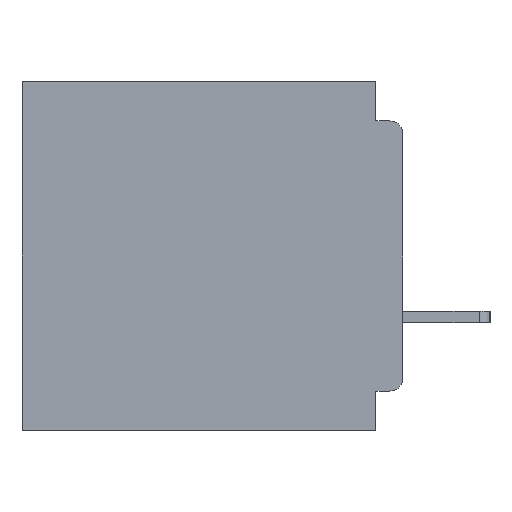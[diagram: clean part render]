
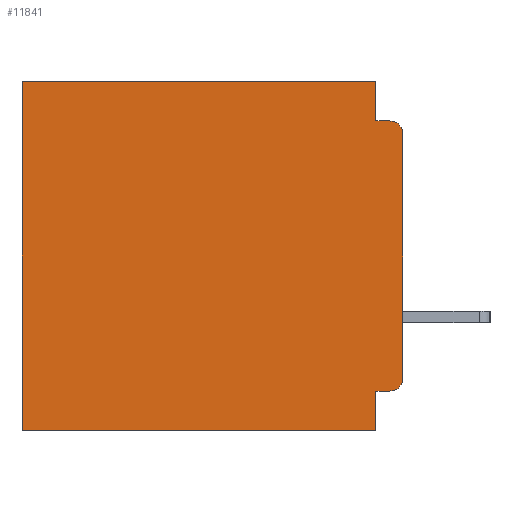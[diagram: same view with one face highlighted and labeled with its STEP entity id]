
A CAD part, left-side view. The second image highlights one B-rep face of the part: STEP entity #11841.
In plain terms, the highlighted planar face has unit normal (-1, 0, 0).
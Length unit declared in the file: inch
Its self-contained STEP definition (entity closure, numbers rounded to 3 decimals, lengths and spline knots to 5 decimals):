
#1046 = LINE ( 'NONE', #38750, #51141 ) ;
#1846 = CARTESIAN_POINT ( 'NONE',  ( 0.3, 0., -0.34 ) ) ;
#1952 = VERTEX_POINT ( 'NONE', #1846 ) ;
#2390 = ORIENTED_EDGE ( 'NONE', *, *, #43696, .T. ) ;
#2711 = ORIENTED_EDGE ( 'NONE', *, *, #8843, .F. ) ;
#3593 = VECTOR ( 'NONE', #11787, 39.37008 ) ;
#4501 = ORIENTED_EDGE ( 'NONE', *, *, #10820, .F. ) ;
#4968 = VERTEX_POINT ( 'NONE', #35830 ) ;
#4974 = EDGE_CURVE ( 'NONE', #32501, #1952, #7253, .T. ) ;
#5276 = ORIENTED_EDGE ( 'NONE', *, *, #4974, .F. ) ;
#5565 = CARTESIAN_POINT ( 'NONE',  ( 0.3, 0.031, -0.4 ) ) ;
#7253 = LINE ( 'NONE', #8095, #28355 ) ;
#7737 = CARTESIAN_POINT ( 'NONE',  ( 0.3, 0., -0.355 ) ) ;
#8095 = CARTESIAN_POINT ( 'NONE',  ( 0.3, 0., -0.4 ) ) ;
#8452 = EDGE_CURVE ( 'NONE', #32501, #28695, #13776, .T. ) ;
#8843 = EDGE_CURVE ( 'NONE', #15329, #44103, #26704, .T. ) ;
#9590 = CARTESIAN_POINT ( 'NONE',  ( 0.3, 0.437, -0.4 ) ) ;
#9704 = DIRECTION ( 'NONE',  ( 0., 1., 0. ) ) ;
#9792 = ORIENTED_EDGE ( 'NONE', *, *, #42569, .T. ) ;
#10611 = DIRECTION ( 'NONE',  ( 0., -1., 0. ) ) ;
#10820 = EDGE_CURVE ( 'NONE', #35454, #15329, #28352, .T. ) ;
#11787 = DIRECTION ( 'NONE',  ( 0., 1., 0. ) ) ;
#11841 = ADVANCED_FACE ( 'NONE', ( #50920 ), #15832, .F. ) ;
#12145 = DIRECTION ( 'NONE',  ( 0., 0., -1. ) ) ;
#13776 = CIRCLE ( 'NONE', #24136, 0.015 ) ;
#14290 = CIRCLE ( 'NONE', #14782, 0.015 ) ;
#14482 = DIRECTION ( 'NONE',  ( -1., 0., 0. ) ) ;
#14782 = AXIS2_PLACEMENT_3D ( 'NONE', #38891, #15288, #42840 ) ;
#14791 = ORIENTED_EDGE ( 'NONE', *, *, #27732, .F. ) ;
#14882 = EDGE_CURVE ( 'NONE', #40064, #35454, #35280, .T. ) ;
#15288 = DIRECTION ( 'NONE',  ( -1., 0., 0. ) ) ;
#15329 = VERTEX_POINT ( 'NONE', #18006 ) ;
#15335 = VECTOR ( 'NONE', #9704, 39.37008 ) ;
#15832 = PLANE ( 'NONE',  #17653 ) ;
#16653 = VECTOR ( 'NONE', #25360, 39.37008 ) ;
#17495 = VECTOR ( 'NONE', #40599, 39.37008 ) ;
#17653 = AXIS2_PLACEMENT_3D ( 'NONE', #27513, #51171, #27692 ) ;
#18006 = CARTESIAN_POINT ( 'NONE',  ( 0.3, 0.031, -0.4 ) ) ;
#19764 = ORIENTED_EDGE ( 'NONE', *, *, #47376, .F. ) ;
#19780 = CARTESIAN_POINT ( 'NONE',  ( 0.3, 0.031, -0.355 ) ) ;
#20289 = LINE ( 'NONE', #32781, #38764 ) ;
#24136 = AXIS2_PLACEMENT_3D ( 'NONE', #38087, #14482, #42040 ) ;
#25360 = DIRECTION ( 'NONE',  ( 0., 0., -1. ) ) ;
#26319 = ORIENTED_EDGE ( 'NONE', *, *, #14882, .F. ) ;
#26677 = EDGE_LOOP ( 'NONE', ( #5276, #44292, #14791, #19764, #9792, #2390, #2711, #4501, #26319, #32527 ) ) ;
#26704 = LINE ( 'NONE', #36692, #17495 ) ;
#26763 = LINE ( 'NONE', #42014, #45208 ) ;
#27513 = CARTESIAN_POINT ( 'NONE',  ( 0.3, 0., -0.4 ) ) ;
#27692 = DIRECTION ( 'NONE',  ( 0., 0., -1. ) ) ;
#27732 = EDGE_CURVE ( 'NONE', #4968, #28695, #26763, .T. ) ;
#28352 = LINE ( 'NONE', #5565, #16653 ) ;
#28355 = VECTOR ( 'NONE', #12145, 39.37008 ) ;
#28695 = VERTEX_POINT ( 'NONE', #32836 ) ;
#29425 = CARTESIAN_POINT ( 'NONE',  ( 0.3, 0., 0. ) ) ;
#30719 = VERTEX_POINT ( 'NONE', #50224 ) ;
#32501 = VERTEX_POINT ( 'NONE', #41996 ) ;
#32527 = ORIENTED_EDGE ( 'NONE', *, *, #33553, .T. ) ;
#32781 = CARTESIAN_POINT ( 'NONE',  ( 0.3, 0.437, -0.4 ) ) ;
#32836 = CARTESIAN_POINT ( 'NONE',  ( 0.3, 0.015, -0.045 ) ) ;
#33553 = EDGE_CURVE ( 'NONE', #40064, #1952, #14290, .T. ) ;
#35280 = LINE ( 'NONE', #7737, #3593 ) ;
#35454 = VERTEX_POINT ( 'NONE', #19780 ) ;
#35830 = CARTESIAN_POINT ( 'NONE',  ( 0.3, 0.031, -0.045 ) ) ;
#35983 = CARTESIAN_POINT ( 'NONE',  ( 0.3, 0.015, -0.355 ) ) ;
#36230 = VERTEX_POINT ( 'NONE', #36917 ) ;
#36321 = LINE ( 'NONE', #29425, #15335 ) ;
#36692 = CARTESIAN_POINT ( 'NONE',  ( 0.3, 0., -0.4 ) ) ;
#36917 = CARTESIAN_POINT ( 'NONE',  ( 0.3, 0.437, 0. ) ) ;
#38087 = CARTESIAN_POINT ( 'NONE',  ( 0.3, 0.015, -0.06 ) ) ;
#38750 = CARTESIAN_POINT ( 'NONE',  ( 0.3, 0.031, 0. ) ) ;
#38764 = VECTOR ( 'NONE', #48380, 39.37008 ) ;
#38891 = CARTESIAN_POINT ( 'NONE',  ( 0.3, 0.015, -0.34 ) ) ;
#40064 = VERTEX_POINT ( 'NONE', #35983 ) ;
#40599 = DIRECTION ( 'NONE',  ( 0., 1., 0. ) ) ;
#41996 = CARTESIAN_POINT ( 'NONE',  ( 0.3, 0., -0.06 ) ) ;
#42014 = CARTESIAN_POINT ( 'NONE',  ( 0.3, 0., -0.045 ) ) ;
#42040 = DIRECTION ( 'NONE',  ( 0., 0., -1. ) ) ;
#42569 = EDGE_CURVE ( 'NONE', #30719, #36230, #36321, .T. ) ;
#42696 = DIRECTION ( 'NONE',  ( 0., 0., -1. ) ) ;
#42840 = DIRECTION ( 'NONE',  ( 0., 0., -1. ) ) ;
#43696 = EDGE_CURVE ( 'NONE', #36230, #44103, #20289, .T. ) ;
#44103 = VERTEX_POINT ( 'NONE', #9590 ) ;
#44292 = ORIENTED_EDGE ( 'NONE', *, *, #8452, .T. ) ;
#45208 = VECTOR ( 'NONE', #10611, 39.37008 ) ;
#47376 = EDGE_CURVE ( 'NONE', #30719, #4968, #1046, .T. ) ;
#48380 = DIRECTION ( 'NONE',  ( 0., 0., -1. ) ) ;
#50224 = CARTESIAN_POINT ( 'NONE',  ( 0.3, 0.031, 0. ) ) ;
#50920 = FACE_OUTER_BOUND ( 'NONE', #26677, .T. ) ;
#51141 = VECTOR ( 'NONE', #42696, 39.37008 ) ;
#51171 = DIRECTION ( 'NONE',  ( 1., 0., 0. ) ) ;
